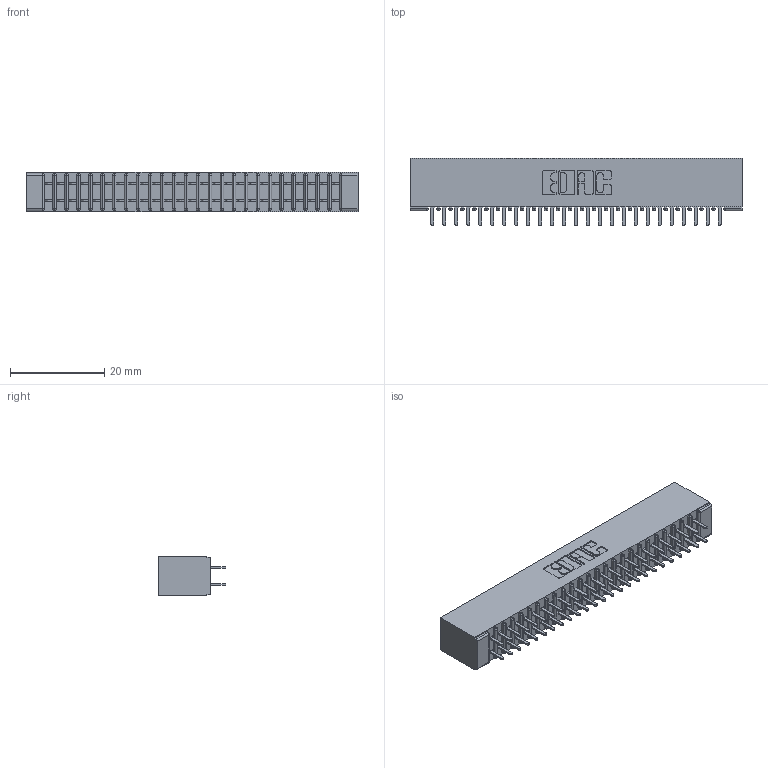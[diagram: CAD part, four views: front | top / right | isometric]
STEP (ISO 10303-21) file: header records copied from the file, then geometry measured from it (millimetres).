
FILE_DESCRIPTION (( 'STEP AP203' ), '1' );
FILE_NAME ('391-050-520-201.STEP', '2018-08-09T04:53:24', ( '' ), ( '' ), 'SwSTEP 2.0', 'SolidWorks 2016', '' );
FILE_SCHEMA (( 'CONFIG_CONTROL_DESIGN' ));
Length unit declared in the file: inch
Products named in the file (3): 341 Part_No Mounting Lugs; 341-292-001_341-292-120; 391-050-520-201
Assembly tree (51 placements, depth 2):
  391-050-520-201
    341 Part_No Mounting Lugs
    341-292-001_341-292-120  x50
Bounding box: 70.48 x 14.27 x 8.38 mm (x, y, z)
Volume: 4135.4 mm3; surface area: 9426.3 mm2
Topology: 51 solids, 51 shells, 3408 faces, 9867 edges, 6390 vertices
Faces by surface type: plane 2064, cylinder 1244, sphere 52, torus 48
Entity records: 32242 total; most frequent: CARTESIAN_POINT 5359, ORIENTED_EDGE 5322, DIRECTION 5211, EDGE_CURVE 2661, LINE 2135, VECTOR 2135, VERTEX_POINT 1686, AXIS2_PLACEMENT_3D 1538
